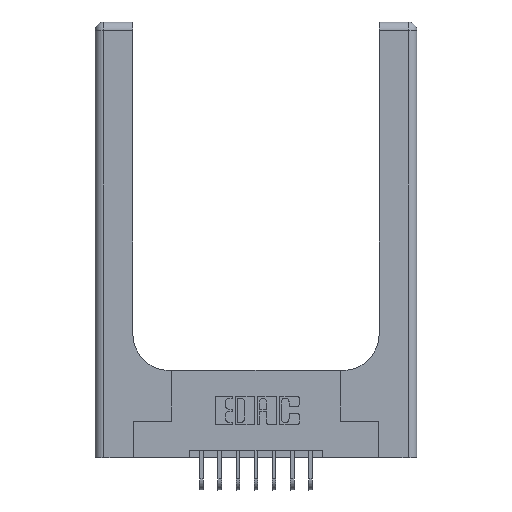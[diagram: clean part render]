
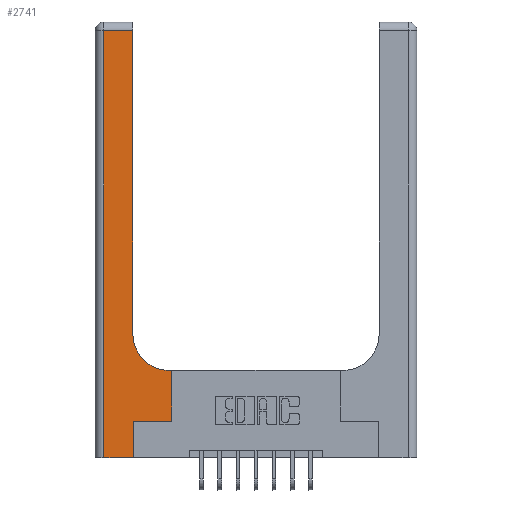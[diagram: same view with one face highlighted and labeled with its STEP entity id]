
A CAD part, top view. The second image highlights one B-rep face of the part: STEP entity #2741.
In plain terms, the highlighted planar face has unit normal (0, 0, 1).
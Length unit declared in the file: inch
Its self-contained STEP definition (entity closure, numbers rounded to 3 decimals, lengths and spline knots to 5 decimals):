
#50 = VECTOR ( 'NONE', #9450, 39.37008 ) ;
#108 = CARTESIAN_POINT ( 'NONE',  ( 0.528, 0.6, 0.37 ) ) ;
#332 = CARTESIAN_POINT ( 'NONE',  ( 0., 2.94, 0.37 ) ) ;
#487 = EDGE_CURVE ( 'NONE', #6303, #16261, #14081, .T. ) ;
#583 = EDGE_CURVE ( 'NONE', #12693, #5366, #6890, .T. ) ;
#605 = CARTESIAN_POINT ( 'NONE',  ( 0.26, 2.94, 0.37 ) ) ;
#726 = VERTEX_POINT ( 'NONE', #605 ) ;
#766 = EDGE_LOOP ( 'NONE', ( #14545, #16405, #11066, #4234, #12932, #6260, #11215, #8511, #10401 ) ) ;
#821 = PLANE ( 'NONE',  #2777 ) ;
#1674 = VECTOR ( 'NONE', #5681, 39.37008 ) ;
#2741 = ADVANCED_FACE ( 'NONE', ( #12396 ), #821, .F. ) ;
#2777 = AXIS2_PLACEMENT_3D ( 'NONE', #3449, #11124, #4721 ) ;
#2832 = CARTESIAN_POINT ( 'NONE',  ( 0.528, 0.25, 0.37 ) ) ;
#3261 = EDGE_CURVE ( 'NONE', #5366, #14512, #5209, .T. ) ;
#3449 = CARTESIAN_POINT ( 'NONE',  ( 0., 3., 0.37 ) ) ;
#3548 = VECTOR ( 'NONE', #3999, 39.37008 ) ;
#3980 = VERTEX_POINT ( 'NONE', #6346 ) ;
#3999 = DIRECTION ( 'NONE',  ( 1., 0., 0. ) ) ;
#4173 = DIRECTION ( 'NONE',  ( 0., 1., 0. ) ) ;
#4234 = ORIENTED_EDGE ( 'NONE', *, *, #6244, .T. ) ;
#4264 = VECTOR ( 'NONE', #16539, 39.37008 ) ;
#4721 = DIRECTION ( 'NONE',  ( -1., 0., 0. ) ) ;
#4738 = DIRECTION ( 'NONE',  ( 0., -1., 0. ) ) ;
#5085 = CARTESIAN_POINT ( 'NONE',  ( 0.26, 3., 0.37 ) ) ;
#5209 = CIRCLE ( 'NONE', #11671, 0.25 ) ;
#5366 = VERTEX_POINT ( 'NONE', #13605 ) ;
#5421 = LINE ( 'NONE', #2832, #15169 ) ;
#5681 = DIRECTION ( 'NONE',  ( 1., 0., 0. ) ) ;
#6244 = EDGE_CURVE ( 'NONE', #3980, #6303, #14991, .T. ) ;
#6260 = ORIENTED_EDGE ( 'NONE', *, *, #8461, .T. ) ;
#6303 = VERTEX_POINT ( 'NONE', #8313 ) ;
#6346 = CARTESIAN_POINT ( 'NONE',  ( 0.06, 0., 0.37 ) ) ;
#6708 = VERTEX_POINT ( 'NONE', #13257 ) ;
#6890 = LINE ( 'NONE', #12020, #12072 ) ;
#7796 = DIRECTION ( 'NONE',  ( 0., 1., 0. ) ) ;
#7812 = EDGE_CURVE ( 'NONE', #13599, #12693, #5421, .T. ) ;
#8313 = CARTESIAN_POINT ( 'NONE',  ( 0.265, 0., 0.37 ) ) ;
#8461 = EDGE_CURVE ( 'NONE', #16261, #13599, #15752, .T. ) ;
#8511 = ORIENTED_EDGE ( 'NONE', *, *, #583, .T. ) ;
#9075 = LINE ( 'NONE', #5085, #12971 ) ;
#9106 = DIRECTION ( 'NONE',  ( 0., 0., -1. ) ) ;
#9450 = DIRECTION ( 'NONE',  ( -1., 0., 0. ) ) ;
#9527 = VECTOR ( 'NONE', #4738, 39.37008 ) ;
#10098 = CARTESIAN_POINT ( 'NONE',  ( 0.528, 0.25, 0.37 ) ) ;
#10300 = CARTESIAN_POINT ( 'NONE',  ( 0.26, 0.85, 0.37 ) ) ;
#10401 = ORIENTED_EDGE ( 'NONE', *, *, #3261, .T. ) ;
#10594 = CARTESIAN_POINT ( 'NONE',  ( 0.265, 0.25, 0.37 ) ) ;
#10595 = EDGE_CURVE ( 'NONE', #14512, #726, #9075, .T. ) ;
#10702 = LINE ( 'NONE', #332, #50 ) ;
#10829 = DIRECTION ( 'NONE',  ( -1., 0., 0. ) ) ;
#11066 = ORIENTED_EDGE ( 'NONE', *, *, #14338, .T. ) ;
#11124 = DIRECTION ( 'NONE',  ( 0., 0., -1. ) ) ;
#11215 = ORIENTED_EDGE ( 'NONE', *, *, #7812, .T. ) ;
#11447 = CARTESIAN_POINT ( 'NONE',  ( 0.265, 0.25, 0.37 ) ) ;
#11510 = CARTESIAN_POINT ( 'NONE',  ( 0., 0., 0.37 ) ) ;
#11671 = AXIS2_PLACEMENT_3D ( 'NONE', #12881, #9106, #14231 ) ;
#12020 = CARTESIAN_POINT ( 'NONE',  ( 0.26, 0.6, 0.37 ) ) ;
#12072 = VECTOR ( 'NONE', #10829, 39.37008 ) ;
#12258 = EDGE_CURVE ( 'NONE', #726, #6708, #10702, .T. ) ;
#12396 = FACE_OUTER_BOUND ( 'NONE', #766, .T. ) ;
#12693 = VERTEX_POINT ( 'NONE', #108 ) ;
#12881 = CARTESIAN_POINT ( 'NONE',  ( 0.51, 0.85, 0.37 ) ) ;
#12932 = ORIENTED_EDGE ( 'NONE', *, *, #487, .T. ) ;
#12971 = VECTOR ( 'NONE', #7796, 39.37008 ) ;
#13257 = CARTESIAN_POINT ( 'NONE',  ( 0.06, 2.94, 0.37 ) ) ;
#13599 = VERTEX_POINT ( 'NONE', #10098 ) ;
#13605 = CARTESIAN_POINT ( 'NONE',  ( 0.51, 0.6, 0.37 ) ) ;
#14081 = LINE ( 'NONE', #14252, #4264 ) ;
#14231 = DIRECTION ( 'NONE',  ( 1., 0., 0. ) ) ;
#14252 = CARTESIAN_POINT ( 'NONE',  ( 0.265, 0., 0.37 ) ) ;
#14338 = EDGE_CURVE ( 'NONE', #6708, #3980, #16307, .T. ) ;
#14512 = VERTEX_POINT ( 'NONE', #10300 ) ;
#14545 = ORIENTED_EDGE ( 'NONE', *, *, #10595, .T. ) ;
#14991 = LINE ( 'NONE', #11510, #3548 ) ;
#15169 = VECTOR ( 'NONE', #4173, 39.37008 ) ;
#15752 = LINE ( 'NONE', #10594, #1674 ) ;
#16261 = VERTEX_POINT ( 'NONE', #11447 ) ;
#16307 = LINE ( 'NONE', #16557, #9527 ) ;
#16405 = ORIENTED_EDGE ( 'NONE', *, *, #12258, .T. ) ;
#16539 = DIRECTION ( 'NONE',  ( 0., 1., 0. ) ) ;
#16557 = CARTESIAN_POINT ( 'NONE',  ( 0.06, 3., 0.37 ) ) ;
